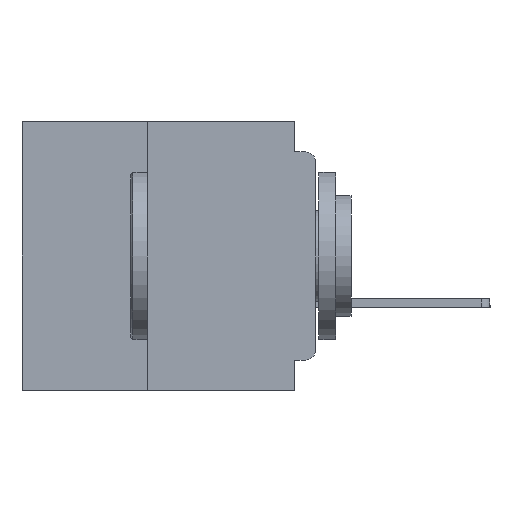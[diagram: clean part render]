
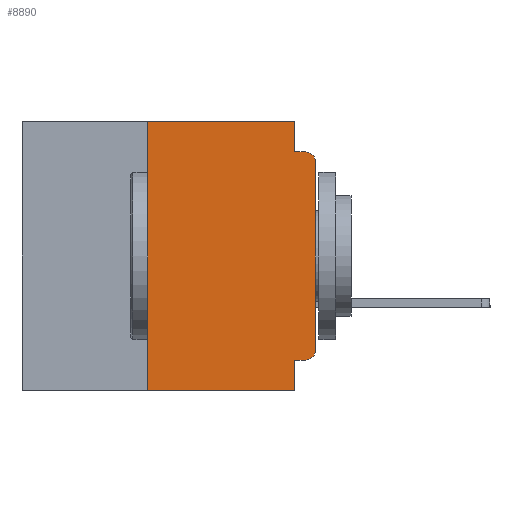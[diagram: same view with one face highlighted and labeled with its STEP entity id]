
A CAD part, left-side view. The second image highlights one B-rep face of the part: STEP entity #8890.
In plain terms, the highlighted planar face has unit normal (-1, 0, 0).
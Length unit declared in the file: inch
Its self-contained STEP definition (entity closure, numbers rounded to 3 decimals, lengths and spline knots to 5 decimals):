
#430 = VERTEX_POINT ( 'NONE', #16803 ) ;
#493 = LINE ( 'NONE', #8478, #34417 ) ;
#1088 = LINE ( 'NONE', #47514, #19836 ) ;
#2331 = CARTESIAN_POINT ( 'NONE',  ( 0., 0.031, 0. ) ) ;
#3486 = AXIS2_PLACEMENT_3D ( 'NONE', #37505, #26375, #3961 ) ;
#3961 = DIRECTION ( 'NONE',  ( 0., 0., -1. ) ) ;
#3975 = ORIENTED_EDGE ( 'NONE', *, *, #15212, .F. ) ;
#4652 = DIRECTION ( 'NONE',  ( 0., 0., -1. ) ) ;
#5221 = ORIENTED_EDGE ( 'NONE', *, *, #21949, .T. ) ;
#5861 = VERTEX_POINT ( 'NONE', #22235 ) ;
#6137 = CARTESIAN_POINT ( 'NONE',  ( 0., 0.25, 0. ) ) ;
#7112 = VECTOR ( 'NONE', #24768, 39.37008 ) ;
#7168 = CARTESIAN_POINT ( 'NONE',  ( 0., 0.015, -0.34 ) ) ;
#7213 = VECTOR ( 'NONE', #33603, 39.37008 ) ;
#8278 = DIRECTION ( 'NONE',  ( 0., 0., 1. ) ) ;
#8478 = CARTESIAN_POINT ( 'NONE',  ( 0., 0.031, -0.4 ) ) ;
#8480 = CARTESIAN_POINT ( 'NONE',  ( 0., 0.437, -0.4 ) ) ;
#8890 = ADVANCED_FACE ( 'NONE', ( #21274 ), #22570, .F. ) ;
#9147 = ORIENTED_EDGE ( 'NONE', *, *, #33966, .F. ) ;
#9703 = ORIENTED_EDGE ( 'NONE', *, *, #16293, .T. ) ;
#9878 = CARTESIAN_POINT ( 'NONE',  ( 0., 0.25, -0.4 ) ) ;
#9945 = CARTESIAN_POINT ( 'NONE',  ( 0., 0.437, 0. ) ) ;
#10866 = EDGE_CURVE ( 'NONE', #45924, #5861, #19330, .T. ) ;
#10958 = DIRECTION ( 'NONE',  ( 0., 0., -1. ) ) ;
#11127 = VECTOR ( 'NONE', #15998, 39.37008 ) ;
#11897 = CARTESIAN_POINT ( 'NONE',  ( 0., 0., 0. ) ) ;
#13208 = ORIENTED_EDGE ( 'NONE', *, *, #27202, .F. ) ;
#14408 = VERTEX_POINT ( 'NONE', #29303 ) ;
#15127 = CIRCLE ( 'NONE', #43673, 0.015 ) ;
#15212 = EDGE_CURVE ( 'NONE', #430, #29194, #1088, .T. ) ;
#15821 = ORIENTED_EDGE ( 'NONE', *, *, #44891, .F. ) ;
#15998 = DIRECTION ( 'NONE',  ( 0., -1., 0. ) ) ;
#16191 = CARTESIAN_POINT ( 'NONE',  ( 0., 0., -0.06 ) ) ;
#16293 = EDGE_CURVE ( 'NONE', #38947, #29194, #36673, .T. ) ;
#16803 = CARTESIAN_POINT ( 'NONE',  ( 0., 0.031, -0.045 ) ) ;
#17096 = CARTESIAN_POINT ( 'NONE',  ( 0., 0.015, -0.06 ) ) ;
#18189 = VECTOR ( 'NONE', #23352, 39.37008 ) ;
#19252 = VERTEX_POINT ( 'NONE', #45599 ) ;
#19330 = LINE ( 'NONE', #38421, #18189 ) ;
#19836 = VECTOR ( 'NONE', #21402, 39.37008 ) ;
#20286 = EDGE_CURVE ( 'NONE', #29385, #30545, #27079, .T. ) ;
#20799 = DIRECTION ( 'NONE',  ( 0., 0., -1. ) ) ;
#21274 = FACE_OUTER_BOUND ( 'NONE', #26621, .T. ) ;
#21402 = DIRECTION ( 'NONE',  ( 0., -1., 0. ) ) ;
#21949 = EDGE_CURVE ( 'NONE', #19252, #38947, #25699, .T. ) ;
#22235 = CARTESIAN_POINT ( 'NONE',  ( 0., 0.031, -0.355 ) ) ;
#22570 = PLANE ( 'NONE',  #3486 ) ;
#23057 = EDGE_CURVE ( 'NONE', #45924, #19252, #15127, .T. ) ;
#23352 = DIRECTION ( 'NONE',  ( 0., 1., 0. ) ) ;
#24768 = DIRECTION ( 'NONE',  ( 0., -1., 0. ) ) ;
#25328 = CARTESIAN_POINT ( 'NONE',  ( 0., 0.015, -0.355 ) ) ;
#25699 = LINE ( 'NONE', #11897, #34481 ) ;
#25829 = VECTOR ( 'NONE', #47104, 39.37008 ) ;
#26072 = CARTESIAN_POINT ( 'NONE',  ( 0., 0.25, -0.4 ) ) ;
#26375 = DIRECTION ( 'NONE',  ( 1., 0., 0. ) ) ;
#26621 = EDGE_LOOP ( 'NONE', ( #5221, #9703, #3975, #9147, #13208, #35259, #27607, #15821, #33425, #27448 ) ) ;
#27079 = LINE ( 'NONE', #26072, #7213 ) ;
#27202 = EDGE_CURVE ( 'NONE', #30545, #14408, #36940, .T. ) ;
#27448 = ORIENTED_EDGE ( 'NONE', *, *, #23057, .T. ) ;
#27607 = ORIENTED_EDGE ( 'NONE', *, *, #37632, .T. ) ;
#29194 = VERTEX_POINT ( 'NONE', #42249 ) ;
#29303 = CARTESIAN_POINT ( 'NONE',  ( 0., 0.031, 0. ) ) ;
#29385 = VERTEX_POINT ( 'NONE', #9878 ) ;
#29959 = CARTESIAN_POINT ( 'NONE',  ( 0., 0.031, -0.4 ) ) ;
#30545 = VERTEX_POINT ( 'NONE', #6137 ) ;
#33305 = DIRECTION ( 'NONE',  ( -1., 0., 0. ) ) ;
#33425 = ORIENTED_EDGE ( 'NONE', *, *, #10866, .F. ) ;
#33603 = DIRECTION ( 'NONE',  ( 0., 0., 1. ) ) ;
#33966 = EDGE_CURVE ( 'NONE', #14408, #430, #45711, .T. ) ;
#34417 = VECTOR ( 'NONE', #4652, 39.37008 ) ;
#34481 = VECTOR ( 'NONE', #8278, 39.37008 ) ;
#35259 = ORIENTED_EDGE ( 'NONE', *, *, #20286, .F. ) ;
#36673 = CIRCLE ( 'NONE', #45303, 0.015 ) ;
#36940 = LINE ( 'NONE', #9945, #7112 ) ;
#37505 = CARTESIAN_POINT ( 'NONE',  ( 0., 0.437, 0. ) ) ;
#37632 = EDGE_CURVE ( 'NONE', #29385, #43643, #40922, .T. ) ;
#38421 = CARTESIAN_POINT ( 'NONE',  ( 0., 0., -0.355 ) ) ;
#38947 = VERTEX_POINT ( 'NONE', #16191 ) ;
#40922 = LINE ( 'NONE', #8480, #11127 ) ;
#42249 = CARTESIAN_POINT ( 'NONE',  ( 0., 0.015, -0.045 ) ) ;
#43210 = DIRECTION ( 'NONE',  ( -1., 0., 0. ) ) ;
#43643 = VERTEX_POINT ( 'NONE', #29959 ) ;
#43673 = AXIS2_PLACEMENT_3D ( 'NONE', #7168, #33305, #10958 ) ;
#44891 = EDGE_CURVE ( 'NONE', #5861, #43643, #493, .T. ) ;
#45303 = AXIS2_PLACEMENT_3D ( 'NONE', #17096, #43210, #20799 ) ;
#45599 = CARTESIAN_POINT ( 'NONE',  ( 0., 0., -0.34 ) ) ;
#45711 = LINE ( 'NONE', #2331, #25829 ) ;
#45924 = VERTEX_POINT ( 'NONE', #25328 ) ;
#47104 = DIRECTION ( 'NONE',  ( 0., 0., -1. ) ) ;
#47514 = CARTESIAN_POINT ( 'NONE',  ( 0., 0., -0.045 ) ) ;
